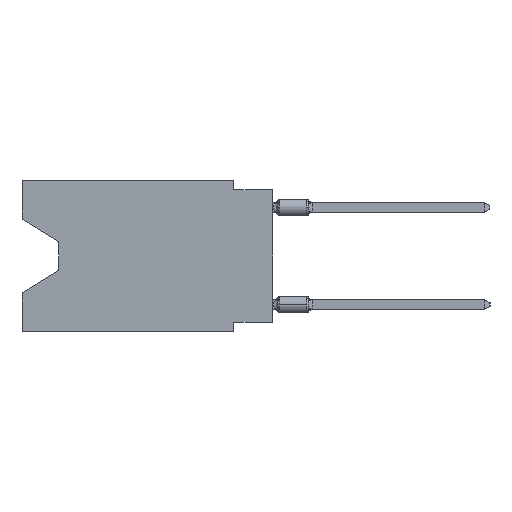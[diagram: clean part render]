
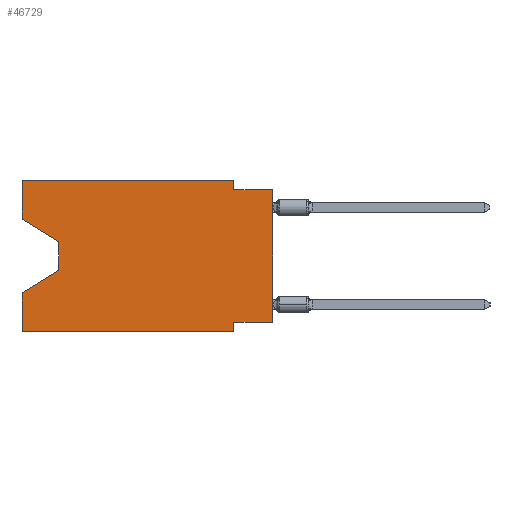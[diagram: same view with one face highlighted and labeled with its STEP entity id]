
A CAD part, left-side view. The second image highlights one B-rep face of the part: STEP entity #46729.
In plain terms, the highlighted planar face has unit normal (-1, 0, 0).
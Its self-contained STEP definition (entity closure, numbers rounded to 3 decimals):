
#252 = CARTESIAN_POINT ( 'NONE',  ( 0., 2.54, -0.635 ) ) ;
#1835 = VECTOR ( 'NONE', #11056, 1000. ) ;
#3264 = CARTESIAN_POINT ( 'NONE',  ( 0., 16.383, -7.36 ) ) ;
#3912 = EDGE_LOOP ( 'NONE', ( #26813, #13241, #7232, #34634, #27767, #23467, #34339, #33835, #6587, #24331, #45363, #13801 ) ) ;
#4471 = DIRECTION ( 'NONE',  ( 0., 0., -1. ) ) ;
#4534 = DIRECTION ( 'NONE',  ( 0., -1., 0. ) ) ;
#6587 = ORIENTED_EDGE ( 'NONE', *, *, #6889, .F. ) ;
#6889 = EDGE_CURVE ( 'NONE', #19312, #21388, #29424, .T. ) ;
#7074 = CARTESIAN_POINT ( 'NONE',  ( 0., 0., -9.271 ) ) ;
#7232 = ORIENTED_EDGE ( 'NONE', *, *, #45201, .T. ) ;
#8176 = CARTESIAN_POINT ( 'NONE',  ( 0., 13.97, -4.013 ) ) ;
#8966 = LINE ( 'NONE', #8176, #32369 ) ;
#9224 = LINE ( 'NONE', #37237, #9590 ) ;
#9443 = VECTOR ( 'NONE', #25676, 1000. ) ;
#9561 = CARTESIAN_POINT ( 'NONE',  ( 0., 2.54, -9.906 ) ) ;
#9590 = VECTOR ( 'NONE', #13188, 1000. ) ;
#10327 = VECTOR ( 'NONE', #27163, 1000. ) ;
#10359 = EDGE_CURVE ( 'NONE', #48221, #43496, #21026, .T. ) ;
#11056 = DIRECTION ( 'NONE',  ( 0., 1., 0. ) ) ;
#11787 = LINE ( 'NONE', #51928, #19448 ) ;
#12329 = VERTEX_POINT ( 'NONE', #15412 ) ;
#12373 = EDGE_CURVE ( 'NONE', #46934, #39586, #32831, .T. ) ;
#12478 = CARTESIAN_POINT ( 'NONE',  ( 0., 16.383, 0. ) ) ;
#13188 = DIRECTION ( 'NONE',  ( 0., 0.855, -0.519 ) ) ;
#13241 = ORIENTED_EDGE ( 'NONE', *, *, #44969, .T. ) ;
#13801 = ORIENTED_EDGE ( 'NONE', *, *, #31028, .F. ) ;
#14658 = CARTESIAN_POINT ( 'NONE',  ( 0., 16.383, -9.906 ) ) ;
#15011 = CARTESIAN_POINT ( 'NONE',  ( 0., 16.383, -9.906 ) ) ;
#15412 = CARTESIAN_POINT ( 'NONE',  ( 0., 13.97, -5.893 ) ) ;
#19312 = VERTEX_POINT ( 'NONE', #252 ) ;
#19448 = VECTOR ( 'NONE', #47202, 1000. ) ;
#19649 = VECTOR ( 'NONE', #4534, 1000. ) ;
#20661 = VERTEX_POINT ( 'NONE', #50117 ) ;
#21026 = LINE ( 'NONE', #32420, #28771 ) ;
#21197 = VERTEX_POINT ( 'NONE', #31746 ) ;
#21388 = VERTEX_POINT ( 'NONE', #32261 ) ;
#22479 = EDGE_CURVE ( 'NONE', #20661, #21388, #36024, .T. ) ;
#23467 = ORIENTED_EDGE ( 'NONE', *, *, #44763, .F. ) ;
#23739 = CARTESIAN_POINT ( 'NONE',  ( 0., 13.97, -4.013 ) ) ;
#23989 = DIRECTION ( 'NONE',  ( 1., 0., 0. ) ) ;
#24331 = ORIENTED_EDGE ( 'NONE', *, *, #27797, .F. ) ;
#25459 = DIRECTION ( 'NONE',  ( 0., -1., 0. ) ) ;
#25676 = DIRECTION ( 'NONE',  ( 0., 0., -1. ) ) ;
#26813 = ORIENTED_EDGE ( 'NONE', *, *, #35411, .T. ) ;
#27160 = LINE ( 'NONE', #47747, #34405 ) ;
#27163 = DIRECTION ( 'NONE',  ( 0., -1., 0. ) ) ;
#27767 = ORIENTED_EDGE ( 'NONE', *, *, #32942, .T. ) ;
#27797 = EDGE_CURVE ( 'NONE', #39586, #19312, #27160, .T. ) ;
#27830 = DIRECTION ( 'NONE',  ( 0., 0., 1. ) ) ;
#27948 = CARTESIAN_POINT ( 'NONE',  ( 0., 16.383, 0. ) ) ;
#28128 = AXIS2_PLACEMENT_3D ( 'NONE', #27948, #23989, #41161 ) ;
#28547 = DIRECTION ( 'NONE',  ( 0., -0.855, -0.519 ) ) ;
#28732 = PLANE ( 'NONE',  #28128 ) ;
#28771 = VECTOR ( 'NONE', #40871, 1000. ) ;
#29424 = LINE ( 'NONE', #41842, #31826 ) ;
#29646 = LINE ( 'NONE', #9561, #9443 ) ;
#31028 = EDGE_CURVE ( 'NONE', #37429, #46934, #11787, .T. ) ;
#31746 = CARTESIAN_POINT ( 'NONE',  ( 0., 2.54, -9.906 ) ) ;
#31826 = VECTOR ( 'NONE', #25459, 1000. ) ;
#32010 = CARTESIAN_POINT ( 'NONE',  ( 0., 16.383, -2.546 ) ) ;
#32261 = CARTESIAN_POINT ( 'NONE',  ( 0., 0., -0.635 ) ) ;
#32332 = CARTESIAN_POINT ( 'NONE',  ( 0., 0., 0. ) ) ;
#32369 = VECTOR ( 'NONE', #4471, 1000. ) ;
#32420 = CARTESIAN_POINT ( 'NONE',  ( 0., 16.383, 0. ) ) ;
#32831 = LINE ( 'NONE', #12478, #19649 ) ;
#32942 = EDGE_CURVE ( 'NONE', #48221, #21197, #35101, .T. ) ;
#33751 = CARTESIAN_POINT ( 'NONE',  ( 0., 16.383, 0. ) ) ;
#33835 = ORIENTED_EDGE ( 'NONE', *, *, #22479, .T. ) ;
#33974 = VECTOR ( 'NONE', #28547, 1000. ) ;
#34339 = ORIENTED_EDGE ( 'NONE', *, *, #44073, .F. ) ;
#34405 = VECTOR ( 'NONE', #43277, 1000. ) ;
#34634 = ORIENTED_EDGE ( 'NONE', *, *, #10359, .F. ) ;
#35101 = LINE ( 'NONE', #15011, #10327 ) ;
#35411 = EDGE_CURVE ( 'NONE', #37429, #39009, #40444, .T. ) ;
#36024 = LINE ( 'NONE', #32332, #47179 ) ;
#37237 = CARTESIAN_POINT ( 'NONE',  ( 0., 13.97, -5.893 ) ) ;
#37429 = VERTEX_POINT ( 'NONE', #45434 ) ;
#39009 = VERTEX_POINT ( 'NONE', #23739 ) ;
#39586 = VERTEX_POINT ( 'NONE', #48492 ) ;
#40372 = FACE_OUTER_BOUND ( 'NONE', #3912, .T. ) ;
#40444 = LINE ( 'NONE', #32010, #33974 ) ;
#40871 = DIRECTION ( 'NONE',  ( 0., 0., 1. ) ) ;
#41161 = DIRECTION ( 'NONE',  ( 0., 0., -1. ) ) ;
#41842 = CARTESIAN_POINT ( 'NONE',  ( 0., 0., -0.635 ) ) ;
#43277 = DIRECTION ( 'NONE',  ( 0., 0., -1. ) ) ;
#43496 = VERTEX_POINT ( 'NONE', #3264 ) ;
#44073 = EDGE_CURVE ( 'NONE', #20661, #45878, #47235, .T. ) ;
#44763 = EDGE_CURVE ( 'NONE', #45878, #21197, #29646, .T. ) ;
#44969 = EDGE_CURVE ( 'NONE', #39009, #12329, #8966, .T. ) ;
#45201 = EDGE_CURVE ( 'NONE', #12329, #43496, #9224, .T. ) ;
#45363 = ORIENTED_EDGE ( 'NONE', *, *, #12373, .F. ) ;
#45434 = CARTESIAN_POINT ( 'NONE',  ( 0., 16.383, -2.546 ) ) ;
#45878 = VERTEX_POINT ( 'NONE', #51914 ) ;
#46729 = ADVANCED_FACE ( 'NONE', ( #40372 ), #28732, .F. ) ;
#46934 = VERTEX_POINT ( 'NONE', #33751 ) ;
#47179 = VECTOR ( 'NONE', #27830, 1000. ) ;
#47202 = DIRECTION ( 'NONE',  ( 0., 0., 1. ) ) ;
#47235 = LINE ( 'NONE', #7074, #1835 ) ;
#47747 = CARTESIAN_POINT ( 'NONE',  ( 0., 2.54, 0. ) ) ;
#48221 = VERTEX_POINT ( 'NONE', #14658 ) ;
#48492 = CARTESIAN_POINT ( 'NONE',  ( 0., 2.54, 0. ) ) ;
#50117 = CARTESIAN_POINT ( 'NONE',  ( 0., 0., -9.271 ) ) ;
#51914 = CARTESIAN_POINT ( 'NONE',  ( 0., 2.54, -9.271 ) ) ;
#51928 = CARTESIAN_POINT ( 'NONE',  ( 0., 16.383, 0. ) ) ;
